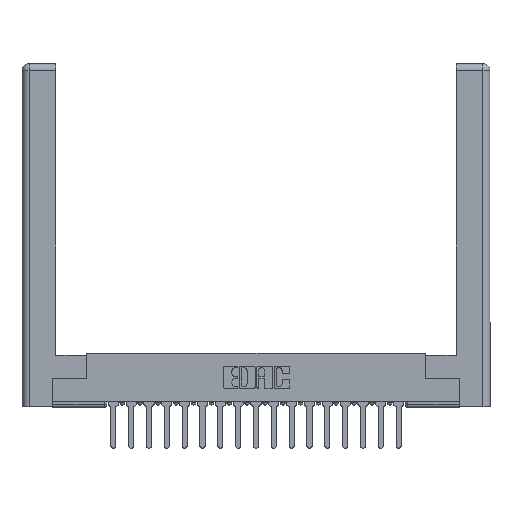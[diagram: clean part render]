
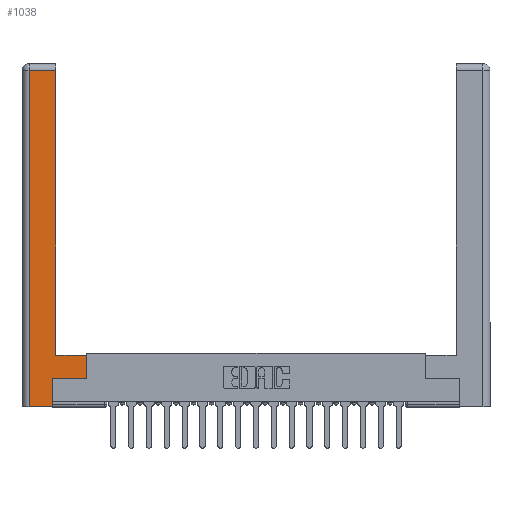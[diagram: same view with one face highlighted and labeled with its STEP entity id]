
A CAD part, top view. The second image highlights one B-rep face of the part: STEP entity #1038.
In plain terms, the highlighted planar face has unit normal (0, 0, 1).
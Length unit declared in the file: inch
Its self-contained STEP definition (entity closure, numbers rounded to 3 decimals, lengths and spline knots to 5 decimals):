
#439 = VERTEX_POINT ( 'NONE', #1469 ) ;
#584 = CARTESIAN_POINT ( 'NONE',  ( 0.0615, 2.94, 0. ) ) ;
#1038 = ADVANCED_FACE ( 'NONE', ( #9733 ), #9929, .F. ) ;
#1392 = ORIENTED_EDGE ( 'NONE', *, *, #18491, .T. ) ;
#1393 = DIRECTION ( 'NONE',  ( -1., 0., 0. ) ) ;
#1433 = ORIENTED_EDGE ( 'NONE', *, *, #17107, .T. ) ;
#1469 = CARTESIAN_POINT ( 'NONE',  ( 0.295, 0.45, 0. ) ) ;
#1472 = EDGE_CURVE ( 'NONE', #439, #1524, #5189, .T. ) ;
#1524 = VERTEX_POINT ( 'NONE', #1922 ) ;
#1715 = DIRECTION ( 'NONE',  ( 0., 1., 0. ) ) ;
#1851 = DIRECTION ( 'NONE',  ( -1., 0., 0. ) ) ;
#1922 = CARTESIAN_POINT ( 'NONE',  ( 0.295, 2.94, 0. ) ) ;
#1946 = CARTESIAN_POINT ( 'NONE',  ( 0., 0., 0. ) ) ;
#4006 = EDGE_LOOP ( 'NONE', ( #20121, #14233, #18962, #19060, #1433, #1392, #7412, #5689 ) ) ;
#4253 = DIRECTION ( 'NONE',  ( 0., 1., 0. ) ) ;
#4448 = EDGE_CURVE ( 'NONE', #14458, #439, #5794, .T. ) ;
#4475 = CARTESIAN_POINT ( 'NONE',  ( 0.295, 0.45, 0. ) ) ;
#4515 = EDGE_CURVE ( 'NONE', #10921, #13282, #16774, .T. ) ;
#5189 = LINE ( 'NONE', #17517, #8247 ) ;
#5312 = EDGE_CURVE ( 'NONE', #16763, #10921, #8621, .T. ) ;
#5647 = CARTESIAN_POINT ( 'NONE',  ( 0.565, 0.245, 0. ) ) ;
#5689 = ORIENTED_EDGE ( 'NONE', *, *, #4448, .T. ) ;
#5784 = LINE ( 'NONE', #18303, #12590 ) ;
#5794 = LINE ( 'NONE', #4475, #6562 ) ;
#6562 = VECTOR ( 'NONE', #1393, 39.37008 ) ;
#6645 = VERTEX_POINT ( 'NONE', #5647 ) ;
#6653 = DIRECTION ( 'NONE',  ( 0., 0., -1. ) ) ;
#7181 = CARTESIAN_POINT ( 'NONE',  ( 0.0615, 0., 0. ) ) ;
#7412 = ORIENTED_EDGE ( 'NONE', *, *, #17299, .T. ) ;
#7599 = AXIS2_PLACEMENT_3D ( 'NONE', #1946, #6653, #1851 ) ;
#8247 = VECTOR ( 'NONE', #1715, 39.37008 ) ;
#8621 = LINE ( 'NONE', #14877, #16097 ) ;
#8709 = CARTESIAN_POINT ( 'NONE',  ( 0.265, 0.245, 0. ) ) ;
#8766 = CARTESIAN_POINT ( 'NONE',  ( 0.565, 0.45, 0. ) ) ;
#8862 = CARTESIAN_POINT ( 'NONE',  ( 0.265, 0., 0. ) ) ;
#9733 = FACE_OUTER_BOUND ( 'NONE', #4006, .T. ) ;
#9929 = PLANE ( 'NONE',  #7599 ) ;
#9993 = LINE ( 'NONE', #584, #15135 ) ;
#10921 = VERTEX_POINT ( 'NONE', #7181 ) ;
#11299 = LINE ( 'NONE', #14380, #17845 ) ;
#11783 = DIRECTION ( 'NONE',  ( 0., -1., 0. ) ) ;
#12272 = VERTEX_POINT ( 'NONE', #8709 ) ;
#12590 = VECTOR ( 'NONE', #4253, 39.37008 ) ;
#13282 = VERTEX_POINT ( 'NONE', #13655 ) ;
#13655 = CARTESIAN_POINT ( 'NONE',  ( 0.265, 0., 0. ) ) ;
#13806 = CARTESIAN_POINT ( 'NONE',  ( 0.0615, 2.94, 0. ) ) ;
#14233 = ORIENTED_EDGE ( 'NONE', *, *, #14341, .T. ) ;
#14341 = EDGE_CURVE ( 'NONE', #1524, #16763, #9993, .T. ) ;
#14380 = CARTESIAN_POINT ( 'NONE',  ( 0.565, 0.45, 0. ) ) ;
#14458 = VERTEX_POINT ( 'NONE', #8766 ) ;
#14877 = CARTESIAN_POINT ( 'NONE',  ( 0.0615, 0., 0. ) ) ;
#15128 = DIRECTION ( 'NONE',  ( 1., 0., 0. ) ) ;
#15135 = VECTOR ( 'NONE', #16366, 39.37008 ) ;
#15636 = DIRECTION ( 'NONE',  ( 1., 0., 0. ) ) ;
#15940 = DIRECTION ( 'NONE',  ( 0., 1., 0. ) ) ;
#16097 = VECTOR ( 'NONE', #11783, 39.37008 ) ;
#16366 = DIRECTION ( 'NONE',  ( -1., 0., 0. ) ) ;
#16550 = VECTOR ( 'NONE', #15636, 39.37008 ) ;
#16763 = VERTEX_POINT ( 'NONE', #13806 ) ;
#16774 = LINE ( 'NONE', #8862, #18036 ) ;
#17107 = EDGE_CURVE ( 'NONE', #13282, #12272, #5784, .T. ) ;
#17183 = LINE ( 'NONE', #18708, #16550 ) ;
#17299 = EDGE_CURVE ( 'NONE', #6645, #14458, #11299, .T. ) ;
#17517 = CARTESIAN_POINT ( 'NONE',  ( 0.295, 3., 0. ) ) ;
#17845 = VECTOR ( 'NONE', #15940, 39.37008 ) ;
#18036 = VECTOR ( 'NONE', #15128, 39.37008 ) ;
#18303 = CARTESIAN_POINT ( 'NONE',  ( 0.265, 0.245, 0. ) ) ;
#18491 = EDGE_CURVE ( 'NONE', #12272, #6645, #17183, .T. ) ;
#18708 = CARTESIAN_POINT ( 'NONE',  ( 0.565, 0.245, 0. ) ) ;
#18962 = ORIENTED_EDGE ( 'NONE', *, *, #5312, .T. ) ;
#19060 = ORIENTED_EDGE ( 'NONE', *, *, #4515, .T. ) ;
#20121 = ORIENTED_EDGE ( 'NONE', *, *, #1472, .T. ) ;
